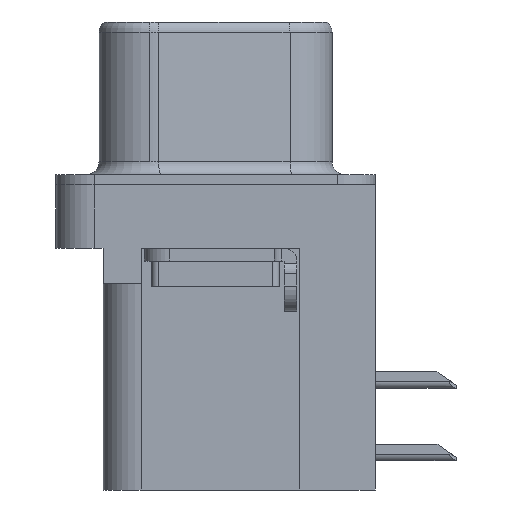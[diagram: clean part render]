
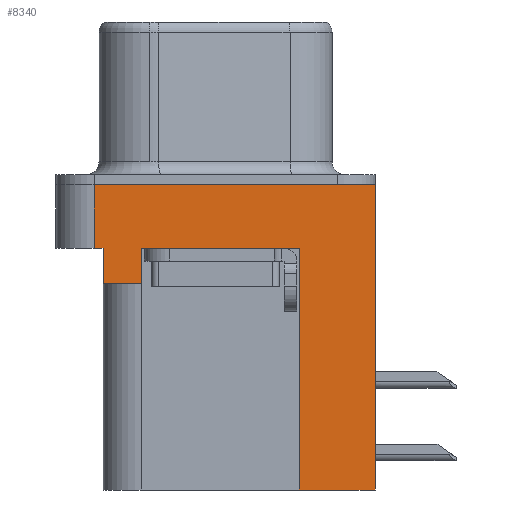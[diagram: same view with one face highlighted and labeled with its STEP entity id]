
A CAD part, left-side view. The second image highlights one B-rep face of the part: STEP entity #8340.
In plain terms, the highlighted planar face has unit normal (-1, 0, 0).
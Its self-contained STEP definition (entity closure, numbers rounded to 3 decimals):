
#745 = ORIENTED_EDGE ( 'NONE', *, *, #6892, .T. ) ;
#931 = CARTESIAN_POINT ( 'NONE',  ( -2.935, -6.275, 0. ) ) ;
#1018 = VERTEX_POINT ( 'NONE', #13312 ) ;
#1797 = CARTESIAN_POINT ( 'NONE',  ( -2.935, 4.775, -2.5 ) ) ;
#2118 = FACE_OUTER_BOUND ( 'NONE', #12230, .T. ) ;
#2163 = ORIENTED_EDGE ( 'NONE', *, *, #7785, .F. ) ;
#2563 = CARTESIAN_POINT ( 'NONE',  ( -2.935, -3.295, -12. ) ) ;
#2598 = CARTESIAN_POINT ( 'NONE',  ( -2.935, -6.275, -2.5 ) ) ;
#2742 = CARTESIAN_POINT ( 'NONE',  ( -2.935, -6.275, 0. ) ) ;
#3444 = ORIENTED_EDGE ( 'NONE', *, *, #7479, .F. ) ;
#3635 = CARTESIAN_POINT ( 'NONE',  ( -2.935, 2.895, -3.9 ) ) ;
#3703 = CARTESIAN_POINT ( 'NONE',  ( -2.935, 4.775, 0. ) ) ;
#3761 = ORIENTED_EDGE ( 'NONE', *, *, #7783, .F. ) ;
#4451 = CARTESIAN_POINT ( 'NONE',  ( -2.935, -3.295, -2.5 ) ) ;
#4862 = VECTOR ( 'NONE', #13029, 1000. ) ;
#4908 = LINE ( 'NONE', #8055, #4862 ) ;
#5040 = VECTOR ( 'NONE', #12930, 1000. ) ;
#5077 = LINE ( 'NONE', #12970, #5117 ) ;
#5117 = VECTOR ( 'NONE', #5243, 1000. ) ;
#5180 = ORIENTED_EDGE ( 'NONE', *, *, #6757, .T. ) ;
#5218 = VECTOR ( 'NONE', #10489, 1000. ) ;
#5243 = DIRECTION ( 'NONE',  ( 0., 0., 1. ) ) ;
#5283 = LINE ( 'NONE', #2563, #5040 ) ;
#5290 = VECTOR ( 'NONE', #6499, 1000. ) ;
#5307 = LINE ( 'NONE', #11654, #5290 ) ;
#5382 = ORIENTED_EDGE ( 'NONE', *, *, #7758, .F. ) ;
#5535 = LINE ( 'NONE', #931, #5710 ) ;
#5672 = VERTEX_POINT ( 'NONE', #15553 ) ;
#5710 = VECTOR ( 'NONE', #6388, 1000. ) ;
#5784 = LINE ( 'NONE', #9244, #5218 ) ;
#5896 = ORIENTED_EDGE ( 'NONE', *, *, #7816, .T. ) ;
#6142 = VECTOR ( 'NONE', #13894, 1000. ) ;
#6332 = LINE ( 'NONE', #9312, #6142 ) ;
#6388 = DIRECTION ( 'NONE',  ( 0., -1., 0. ) ) ;
#6499 = DIRECTION ( 'NONE',  ( 0., 0., 1. ) ) ;
#6595 = CARTESIAN_POINT ( 'NONE',  ( -2.935, -6.275, -12. ) ) ;
#6659 = DIRECTION ( 'NONE',  ( -1., 0., 0. ) ) ;
#6710 = VECTOR ( 'NONE', #8795, 1000. ) ;
#6757 = EDGE_CURVE ( 'NONE', #1018, #9456, #11268, .T. ) ;
#6763 = LINE ( 'NONE', #14527, #6710 ) ;
#6892 = EDGE_CURVE ( 'NONE', #6938, #1018, #10499, .T. ) ;
#6938 = VERTEX_POINT ( 'NONE', #9291 ) ;
#7114 = VERTEX_POINT ( 'NONE', #2742 ) ;
#7479 = EDGE_CURVE ( 'NONE', #6938, #11598, #6763, .T. ) ;
#7524 = CARTESIAN_POINT ( 'NONE',  ( -2.935, 4.425, -2.5 ) ) ;
#7588 = EDGE_CURVE ( 'NONE', #10044, #11660, #6332, .T. ) ;
#7708 = EDGE_CURVE ( 'NONE', #12370, #7114, #5535, .T. ) ;
#7731 = EDGE_CURVE ( 'NONE', #10044, #12370, #5307, .T. ) ;
#7758 = EDGE_CURVE ( 'NONE', #11598, #11660, #5784, .T. ) ;
#7783 = EDGE_CURVE ( 'NONE', #5672, #9456, #5077, .T. ) ;
#7785 = EDGE_CURVE ( 'NONE', #11894, #5672, #5283, .T. ) ;
#7816 = EDGE_CURVE ( 'NONE', #11894, #7114, #4908, .T. ) ;
#8055 = CARTESIAN_POINT ( 'NONE',  ( -2.935, -6.275, -2.5 ) ) ;
#8340 = ADVANCED_FACE ( 'NONE', ( #2118 ), #14207, .T. ) ;
#8659 = ORIENTED_EDGE ( 'NONE', *, *, #7731, .F. ) ;
#8795 = DIRECTION ( 'NONE',  ( 0., 1., 0. ) ) ;
#8973 = ORIENTED_EDGE ( 'NONE', *, *, #7708, .F. ) ;
#9244 = CARTESIAN_POINT ( 'NONE',  ( -2.935, 4.425, -3.9 ) ) ;
#9291 = CARTESIAN_POINT ( 'NONE',  ( -2.935, 2.895, -3.9 ) ) ;
#9312 = CARTESIAN_POINT ( 'NONE',  ( -2.935, -6.275, -2.5 ) ) ;
#9456 = VERTEX_POINT ( 'NONE', #4451 ) ;
#10044 = VERTEX_POINT ( 'NONE', #1797 ) ;
#10421 = ORIENTED_EDGE ( 'NONE', *, *, #7588, .T. ) ;
#10489 = DIRECTION ( 'NONE',  ( 0., 0., 1. ) ) ;
#10499 = LINE ( 'NONE', #3635, #10514 ) ;
#10514 = VECTOR ( 'NONE', #11936, 1000. ) ;
#11227 = VECTOR ( 'NONE', #16083, 1000. ) ;
#11268 = LINE ( 'NONE', #15332, #11227 ) ;
#11598 = VERTEX_POINT ( 'NONE', #14813 ) ;
#11654 = CARTESIAN_POINT ( 'NONE',  ( -2.935, 4.775, -2.5 ) ) ;
#11660 = VERTEX_POINT ( 'NONE', #7524 ) ;
#11894 = VERTEX_POINT ( 'NONE', #6595 ) ;
#11936 = DIRECTION ( 'NONE',  ( 0., 0., 1. ) ) ;
#12230 = EDGE_LOOP ( 'NONE', ( #8973, #8659, #10421, #5382, #3444, #745, #5180, #3761, #2163, #5896 ) ) ;
#12370 = VERTEX_POINT ( 'NONE', #3703 ) ;
#12930 = DIRECTION ( 'NONE',  ( 0., 1., 0. ) ) ;
#12970 = CARTESIAN_POINT ( 'NONE',  ( -2.935, -3.295, -12. ) ) ;
#13029 = DIRECTION ( 'NONE',  ( 0., 0., 1. ) ) ;
#13312 = CARTESIAN_POINT ( 'NONE',  ( -2.935, 2.895, -2.5 ) ) ;
#13894 = DIRECTION ( 'NONE',  ( 0., -1., 0. ) ) ;
#14207 = PLANE ( 'NONE',  #15694 ) ;
#14527 = CARTESIAN_POINT ( 'NONE',  ( -2.935, 4.425, -3.9 ) ) ;
#14813 = CARTESIAN_POINT ( 'NONE',  ( -2.935, 4.425, -3.9 ) ) ;
#15332 = CARTESIAN_POINT ( 'NONE',  ( -2.935, -6.275, -2.5 ) ) ;
#15354 = DIRECTION ( 'NONE',  ( 0., 0., 1. ) ) ;
#15553 = CARTESIAN_POINT ( 'NONE',  ( -2.935, -3.295, -12. ) ) ;
#15694 = AXIS2_PLACEMENT_3D ( 'NONE', #2598, #6659, #15354 ) ;
#16083 = DIRECTION ( 'NONE',  ( 0., -1., 0. ) ) ;
